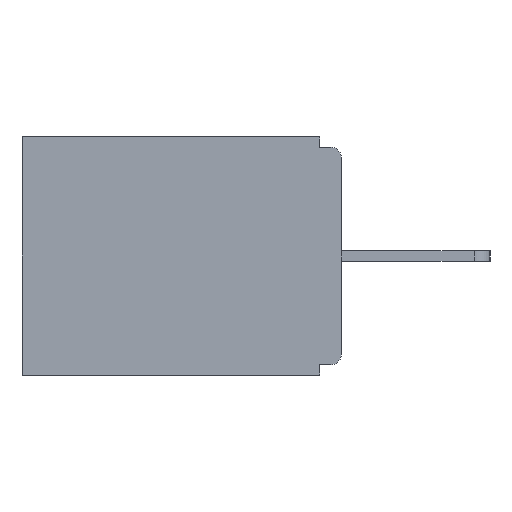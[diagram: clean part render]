
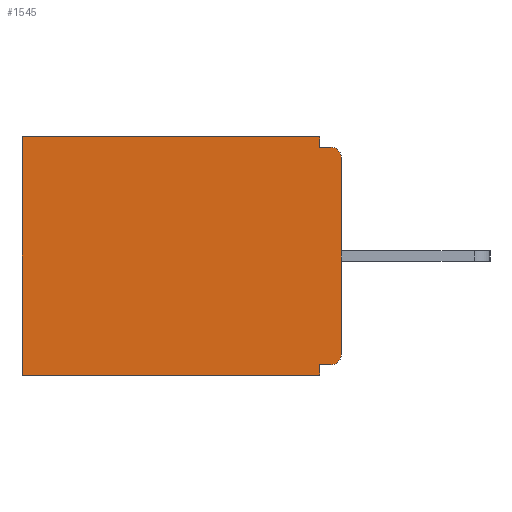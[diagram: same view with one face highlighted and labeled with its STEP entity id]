
A CAD part, left-side view. The second image highlights one B-rep face of the part: STEP entity #1545.
In plain terms, the highlighted planar face has unit normal (-1, 0, 0).
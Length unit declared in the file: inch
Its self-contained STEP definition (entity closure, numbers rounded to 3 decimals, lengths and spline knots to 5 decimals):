
#342 = LINE ( 'NONE', #2814, #5723 ) ;
#454 = EDGE_CURVE ( 'NONE', #6602, #5550, #5635, .T. ) ;
#610 = EDGE_CURVE ( 'NONE', #2096, #10768, #9524, .T. ) ;
#683 = EDGE_CURVE ( 'NONE', #8228, #8089, #2291, .T. ) ;
#830 = EDGE_CURVE ( 'NONE', #2096, #5550, #4533, .T. ) ;
#889 = DIRECTION ( 'NONE',  ( -1., 0., 0. ) ) ;
#928 = EDGE_CURVE ( 'NONE', #6602, #8089, #5614, .T. ) ;
#1117 = DIRECTION ( 'NONE',  ( 0., 0., -1. ) ) ;
#1219 = CARTESIAN_POINT ( 'NONE',  ( 0.298, 0., -0.328 ) ) ;
#1545 = ADVANCED_FACE ( 'NONE', ( #9886 ), #11466, .F. ) ;
#1645 = EDGE_CURVE ( 'NONE', #9794, #6849, #9746, .T. ) ;
#1843 = ORIENTED_EDGE ( 'NONE', *, *, #928, .T. ) ;
#1920 = AXIS2_PLACEMENT_3D ( 'NONE', #10114, #10123, #10773 ) ;
#1937 = CARTESIAN_POINT ( 'NONE',  ( 0.298, 0.031, -0.328 ) ) ;
#2057 = VECTOR ( 'NONE', #7013, 39.37008 ) ;
#2096 = VERTEX_POINT ( 'NONE', #3917 ) ;
#2167 = AXIS2_PLACEMENT_3D ( 'NONE', #9398, #6672, #5651 ) ;
#2291 = LINE ( 'NONE', #6971, #11816 ) ;
#2531 = DIRECTION ( 'NONE',  ( 0., 1., 0. ) ) ;
#2814 = CARTESIAN_POINT ( 'NONE',  ( 0.298, 0.031, -0.343 ) ) ;
#2924 = EDGE_CURVE ( 'NONE', #6278, #8228, #342, .T. ) ;
#2961 = VECTOR ( 'NONE', #4418, 39.37008 ) ;
#3048 = EDGE_CURVE ( 'NONE', #10768, #9794, #7629, .T. ) ;
#3324 = CARTESIAN_POINT ( 'NONE',  ( 0.298, 0.46, 0. ) ) ;
#3742 = EDGE_CURVE ( 'NONE', #12267, #6849, #11415, .T. ) ;
#3749 = DIRECTION ( 'NONE',  ( 0., 0., -1. ) ) ;
#3917 = CARTESIAN_POINT ( 'NONE',  ( 0.298, 0.015, -0.328 ) ) ;
#4010 = AXIS2_PLACEMENT_3D ( 'NONE', #9846, #889, #7349 ) ;
#4418 = DIRECTION ( 'NONE',  ( 0., 0., -1. ) ) ;
#4524 = VECTOR ( 'NONE', #4876, 39.37008 ) ;
#4533 = CIRCLE ( 'NONE', #1920, 0.015 ) ;
#4811 = VECTOR ( 'NONE', #3749, 39.37008 ) ;
#4876 = DIRECTION ( 'NONE',  ( 0., 1., 0. ) ) ;
#5225 = ORIENTED_EDGE ( 'NONE', *, *, #1645, .F. ) ;
#5503 = CARTESIAN_POINT ( 'NONE',  ( 0.298, 0., -0.343 ) ) ;
#5550 = VERTEX_POINT ( 'NONE', #7683 ) ;
#5614 = CIRCLE ( 'NONE', #4010, 0.015 ) ;
#5635 = LINE ( 'NONE', #12044, #2961 ) ;
#5651 = DIRECTION ( 'NONE',  ( 0., 0., -1. ) ) ;
#5723 = VECTOR ( 'NONE', #1117, 39.37008 ) ;
#5750 = CARTESIAN_POINT ( 'NONE',  ( 0.298, 0.46, -0.343 ) ) ;
#6278 = VERTEX_POINT ( 'NONE', #11330 ) ;
#6602 = VERTEX_POINT ( 'NONE', #7278 ) ;
#6672 = DIRECTION ( 'NONE',  ( 1., 0., 0. ) ) ;
#6849 = VERTEX_POINT ( 'NONE', #5750 ) ;
#6971 = CARTESIAN_POINT ( 'NONE',  ( 0.298, 0., -0.015 ) ) ;
#7013 = DIRECTION ( 'NONE',  ( 0., 1., 0. ) ) ;
#7124 = CARTESIAN_POINT ( 'NONE',  ( 0.298, 0.46, 0. ) ) ;
#7278 = CARTESIAN_POINT ( 'NONE',  ( 0.298, 0., -0.03 ) ) ;
#7349 = DIRECTION ( 'NONE',  ( 0., 0., -1. ) ) ;
#7385 = CARTESIAN_POINT ( 'NONE',  ( 0.298, 0.031, -0.343 ) ) ;
#7510 = CARTESIAN_POINT ( 'NONE',  ( 0.298, 0.031, -0.343 ) ) ;
#7629 = LINE ( 'NONE', #7385, #4811 ) ;
#7683 = CARTESIAN_POINT ( 'NONE',  ( 0.298, 0., -0.313 ) ) ;
#7726 = DIRECTION ( 'NONE',  ( 0., 0., -1. ) ) ;
#7946 = LINE ( 'NONE', #11970, #4524 ) ;
#8089 = VERTEX_POINT ( 'NONE', #9902 ) ;
#8228 = VERTEX_POINT ( 'NONE', #10001 ) ;
#8521 = EDGE_CURVE ( 'NONE', #6278, #12267, #7946, .T. ) ;
#9006 = ORIENTED_EDGE ( 'NONE', *, *, #3742, .T. ) ;
#9162 = VECTOR ( 'NONE', #7726, 39.37008 ) ;
#9165 = ORIENTED_EDGE ( 'NONE', *, *, #3048, .F. ) ;
#9286 = ORIENTED_EDGE ( 'NONE', *, *, #8521, .T. ) ;
#9398 = CARTESIAN_POINT ( 'NONE',  ( 0.298, 0., 0. ) ) ;
#9524 = LINE ( 'NONE', #1219, #11706 ) ;
#9746 = LINE ( 'NONE', #5503, #2057 ) ;
#9794 = VERTEX_POINT ( 'NONE', #7510 ) ;
#9846 = CARTESIAN_POINT ( 'NONE',  ( 0.298, 0.015, -0.03 ) ) ;
#9886 = FACE_OUTER_BOUND ( 'NONE', #12085, .T. ) ;
#9902 = CARTESIAN_POINT ( 'NONE',  ( 0.298, 0.015, -0.015 ) ) ;
#10001 = CARTESIAN_POINT ( 'NONE',  ( 0.298, 0.031, -0.015 ) ) ;
#10114 = CARTESIAN_POINT ( 'NONE',  ( 0.298, 0.015, -0.313 ) ) ;
#10123 = DIRECTION ( 'NONE',  ( -1., 0., 0. ) ) ;
#10738 = ORIENTED_EDGE ( 'NONE', *, *, #683, .F. ) ;
#10768 = VERTEX_POINT ( 'NONE', #1937 ) ;
#10773 = DIRECTION ( 'NONE',  ( 0., 0., -1. ) ) ;
#11061 = DIRECTION ( 'NONE',  ( 0., -1., 0. ) ) ;
#11254 = ORIENTED_EDGE ( 'NONE', *, *, #2924, .F. ) ;
#11330 = CARTESIAN_POINT ( 'NONE',  ( 0.298, 0.031, 0. ) ) ;
#11415 = LINE ( 'NONE', #7124, #9162 ) ;
#11466 = PLANE ( 'NONE',  #2167 ) ;
#11472 = ORIENTED_EDGE ( 'NONE', *, *, #454, .F. ) ;
#11706 = VECTOR ( 'NONE', #2531, 39.37008 ) ;
#11711 = ORIENTED_EDGE ( 'NONE', *, *, #830, .T. ) ;
#11816 = VECTOR ( 'NONE', #11061, 39.37008 ) ;
#11821 = ORIENTED_EDGE ( 'NONE', *, *, #610, .F. ) ;
#11970 = CARTESIAN_POINT ( 'NONE',  ( 0.298, 0., 0. ) ) ;
#12044 = CARTESIAN_POINT ( 'NONE',  ( 0.298, 0., 0. ) ) ;
#12085 = EDGE_LOOP ( 'NONE', ( #1843, #10738, #11254, #9286, #9006, #5225, #9165, #11821, #11711, #11472 ) ) ;
#12267 = VERTEX_POINT ( 'NONE', #3324 ) ;
